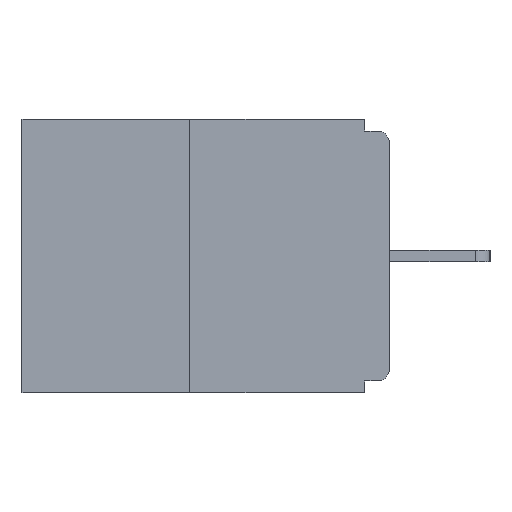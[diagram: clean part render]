
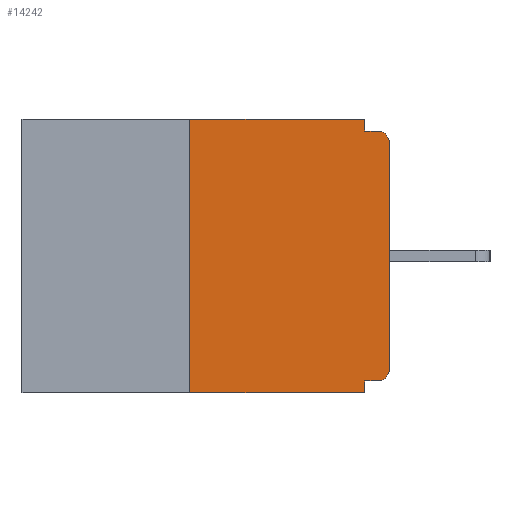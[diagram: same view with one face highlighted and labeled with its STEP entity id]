
A CAD part, left-side view. The second image highlights one B-rep face of the part: STEP entity #14242.
In plain terms, the highlighted planar face has unit normal (-1, 0, 0).
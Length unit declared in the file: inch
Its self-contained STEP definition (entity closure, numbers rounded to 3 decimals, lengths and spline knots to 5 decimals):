
#52 = DIRECTION ( 'NONE',  ( 0., 0., -1. ) ) ;
#213 = EDGE_CURVE ( 'NONE', #14799, #7632, #1364, .T. ) ;
#329 = DIRECTION ( 'NONE',  ( 0., 0., -1. ) ) ;
#610 = CARTESIAN_POINT ( 'NONE',  ( 0., 0.031, -0.343 ) ) ;
#872 = ORIENTED_EDGE ( 'NONE', *, *, #15567, .T. ) ;
#1364 = LINE ( 'NONE', #8742, #15414 ) ;
#1682 = ORIENTED_EDGE ( 'NONE', *, *, #213, .F. ) ;
#1912 = CARTESIAN_POINT ( 'NONE',  ( 0., 0.015, -0.03 ) ) ;
#1992 = CARTESIAN_POINT ( 'NONE',  ( 0., 0.25, -0.343 ) ) ;
#2141 = DIRECTION ( 'NONE',  ( 0., -1., 0. ) ) ;
#2193 = CARTESIAN_POINT ( 'NONE',  ( 0., 0.031, -0.343 ) ) ;
#2347 = VERTEX_POINT ( 'NONE', #1992 ) ;
#2352 = CARTESIAN_POINT ( 'NONE',  ( 0., 0.25, 0. ) ) ;
#2355 = VECTOR ( 'NONE', #10329, 39.37008 ) ;
#2429 = CARTESIAN_POINT ( 'NONE',  ( 0., 0.015, -0.015 ) ) ;
#2614 = CARTESIAN_POINT ( 'NONE',  ( 0., 0.031, -0.015 ) ) ;
#3249 = LINE ( 'NONE', #2193, #2355 ) ;
#3812 = CARTESIAN_POINT ( 'NONE',  ( 0., 0., -0.313 ) ) ;
#4132 = VERTEX_POINT ( 'NONE', #610 ) ;
#4137 = PLANE ( 'NONE',  #14089 ) ;
#4389 = EDGE_CURVE ( 'NONE', #2347, #12089, #11375, .T. ) ;
#4710 = DIRECTION ( 'NONE',  ( 0., 0., -1. ) ) ;
#4781 = DIRECTION ( 'NONE',  ( -1., 0., 0. ) ) ;
#4913 = DIRECTION ( 'NONE',  ( 0., 0., 1. ) ) ;
#5005 = CARTESIAN_POINT ( 'NONE',  ( 0., 0., -0.015 ) ) ;
#5186 = ORIENTED_EDGE ( 'NONE', *, *, #15627, .F. ) ;
#5275 = CARTESIAN_POINT ( 'NONE',  ( 0., 0., -0.03 ) ) ;
#5336 = CARTESIAN_POINT ( 'NONE',  ( 0., 0., -0.328 ) ) ;
#5607 = CARTESIAN_POINT ( 'NONE',  ( 0., 0.015, -0.313 ) ) ;
#5877 = CARTESIAN_POINT ( 'NONE',  ( 0., 0.25, 0. ) ) ;
#5941 = EDGE_CURVE ( 'NONE', #16404, #9381, #17205, .T. ) ;
#6260 = CARTESIAN_POINT ( 'NONE',  ( 0., 0.46, -0.343 ) ) ;
#6393 = CARTESIAN_POINT ( 'NONE',  ( 0., 0., 0. ) ) ;
#6505 = AXIS2_PLACEMENT_3D ( 'NONE', #5607, #6986, #16659 ) ;
#6588 = AXIS2_PLACEMENT_3D ( 'NONE', #1912, #4781, #4710 ) ;
#6986 = DIRECTION ( 'NONE',  ( -1., 0., 0. ) ) ;
#7120 = VECTOR ( 'NONE', #2141, 39.37008 ) ;
#7632 = VERTEX_POINT ( 'NONE', #2614 ) ;
#7715 = DIRECTION ( 'NONE',  ( 0., 0., 1. ) ) ;
#7842 = CARTESIAN_POINT ( 'NONE',  ( 0., 0.46, 0. ) ) ;
#7978 = CIRCLE ( 'NONE', #6505, 0.015 ) ;
#8324 = VECTOR ( 'NONE', #7715, 39.37008 ) ;
#8491 = EDGE_LOOP ( 'NONE', ( #9113, #13466, #12149, #13317, #5186, #10234, #872, #17274, #13210, #1682 ) ) ;
#8742 = CARTESIAN_POINT ( 'NONE',  ( 0., 0.031, 0. ) ) ;
#9113 = ORIENTED_EDGE ( 'NONE', *, *, #15224, .F. ) ;
#9381 = VERTEX_POINT ( 'NONE', #2429 ) ;
#9693 = LINE ( 'NONE', #7842, #11204 ) ;
#10234 = ORIENTED_EDGE ( 'NONE', *, *, #12568, .T. ) ;
#10329 = DIRECTION ( 'NONE',  ( 0., 0., -1. ) ) ;
#10643 = VERTEX_POINT ( 'NONE', #12193 ) ;
#10664 = DIRECTION ( 'NONE',  ( 0., 1., 0. ) ) ;
#10875 = CARTESIAN_POINT ( 'NONE',  ( 0., 0.46, 0. ) ) ;
#11204 = VECTOR ( 'NONE', #16205, 39.37008 ) ;
#11375 = LINE ( 'NONE', #2352, #8324 ) ;
#11774 = EDGE_CURVE ( 'NONE', #2347, #4132, #14507, .T. ) ;
#12089 = VERTEX_POINT ( 'NONE', #5877 ) ;
#12149 = ORIENTED_EDGE ( 'NONE', *, *, #11774, .T. ) ;
#12170 = VERTEX_POINT ( 'NONE', #13073 ) ;
#12193 = CARTESIAN_POINT ( 'NONE',  ( 0., 0.015, -0.328 ) ) ;
#12301 = VECTOR ( 'NONE', #4913, 39.37008 ) ;
#12568 = EDGE_CURVE ( 'NONE', #10643, #15655, #7978, .T. ) ;
#13073 = CARTESIAN_POINT ( 'NONE',  ( 0., 0.031, -0.328 ) ) ;
#13152 = VECTOR ( 'NONE', #17292, 39.37008 ) ;
#13210 = ORIENTED_EDGE ( 'NONE', *, *, #14028, .F. ) ;
#13317 = ORIENTED_EDGE ( 'NONE', *, *, #15119, .F. ) ;
#13466 = ORIENTED_EDGE ( 'NONE', *, *, #4389, .F. ) ;
#13589 = LINE ( 'NONE', #5005, #13152 ) ;
#14028 = EDGE_CURVE ( 'NONE', #7632, #9381, #13589, .T. ) ;
#14037 = LINE ( 'NONE', #6393, #12301 ) ;
#14089 = AXIS2_PLACEMENT_3D ( 'NONE', #10875, #16568, #52 ) ;
#14242 = ADVANCED_FACE ( 'NONE', ( #17632 ), #4137, .F. ) ;
#14507 = LINE ( 'NONE', #6260, #7120 ) ;
#14799 = VERTEX_POINT ( 'NONE', #17555 ) ;
#15119 = EDGE_CURVE ( 'NONE', #12170, #4132, #3249, .T. ) ;
#15224 = EDGE_CURVE ( 'NONE', #12089, #14799, #9693, .T. ) ;
#15414 = VECTOR ( 'NONE', #329, 39.37008 ) ;
#15567 = EDGE_CURVE ( 'NONE', #15655, #16404, #14037, .T. ) ;
#15627 = EDGE_CURVE ( 'NONE', #10643, #12170, #17230, .T. ) ;
#15655 = VERTEX_POINT ( 'NONE', #3812 ) ;
#16205 = DIRECTION ( 'NONE',  ( 0., -1., 0. ) ) ;
#16387 = VECTOR ( 'NONE', #10664, 39.37008 ) ;
#16404 = VERTEX_POINT ( 'NONE', #5275 ) ;
#16568 = DIRECTION ( 'NONE',  ( 1., 0., 0. ) ) ;
#16659 = DIRECTION ( 'NONE',  ( 0., 0., -1. ) ) ;
#17205 = CIRCLE ( 'NONE', #6588, 0.015 ) ;
#17230 = LINE ( 'NONE', #5336, #16387 ) ;
#17274 = ORIENTED_EDGE ( 'NONE', *, *, #5941, .T. ) ;
#17292 = DIRECTION ( 'NONE',  ( 0., -1., 0. ) ) ;
#17555 = CARTESIAN_POINT ( 'NONE',  ( 0., 0.031, 0. ) ) ;
#17632 = FACE_OUTER_BOUND ( 'NONE', #8491, .T. ) ;
